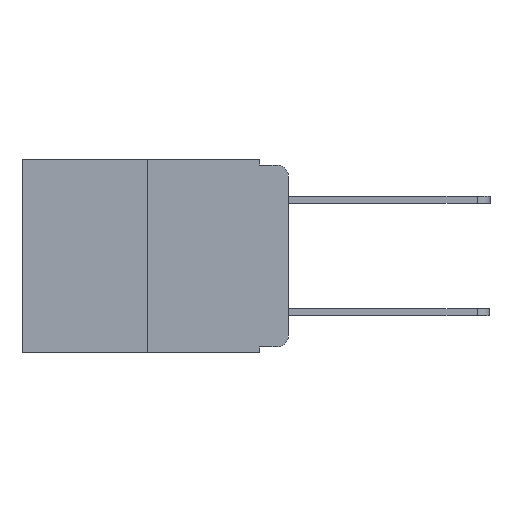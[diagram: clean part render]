
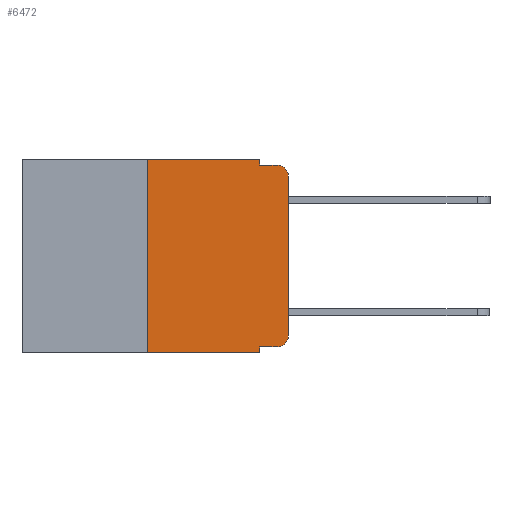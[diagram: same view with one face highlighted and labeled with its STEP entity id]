
A CAD part, left-side view. The second image highlights one B-rep face of the part: STEP entity #6472.
In plain terms, the highlighted planar face has unit normal (-1, 0, 0).
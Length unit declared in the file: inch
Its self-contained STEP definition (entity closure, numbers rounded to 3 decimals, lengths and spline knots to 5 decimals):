
#864 = EDGE_CURVE ( 'NONE', #1789, #5120, #11651, .T. ) ;
#1062 = AXIS2_PLACEMENT_3D ( 'NONE', #12072, #8657, #2610 ) ;
#1295 = ORIENTED_EDGE ( 'NONE', *, *, #1380, .F. ) ;
#1339 = DIRECTION ( 'NONE',  ( 0., -1., 0. ) ) ;
#1380 = EDGE_CURVE ( 'NONE', #1460, #12300, #2654, .T. ) ;
#1411 = ORIENTED_EDGE ( 'NONE', *, *, #11492, .F. ) ;
#1416 = VECTOR ( 'NONE', #6540, 39.37008 ) ;
#1460 = VERTEX_POINT ( 'NONE', #9998 ) ;
#1789 = VERTEX_POINT ( 'NONE', #4084 ) ;
#1919 = ORIENTED_EDGE ( 'NONE', *, *, #5005, .T. ) ;
#2190 = CARTESIAN_POINT ( 'NONE',  ( 0., 0.473, -0.343 ) ) ;
#2516 = ORIENTED_EDGE ( 'NONE', *, *, #864, .F. ) ;
#2531 = DIRECTION ( 'NONE',  ( 0., 0., -1. ) ) ;
#2559 = CIRCLE ( 'NONE', #4141, 0.02 ) ;
#2595 = LINE ( 'NONE', #4048, #12362 ) ;
#2610 = DIRECTION ( 'NONE',  ( 0., 0., -1. ) ) ;
#2654 = LINE ( 'NONE', #3460, #10198 ) ;
#2834 = DIRECTION ( 'NONE',  ( -1., 0., 0. ) ) ;
#2876 = ORIENTED_EDGE ( 'NONE', *, *, #6896, .F. ) ;
#2973 = CARTESIAN_POINT ( 'NONE',  ( 0., 0.051, -0.333 ) ) ;
#3060 = EDGE_LOOP ( 'NONE', ( #8102, #8276, #1411, #3928, #2516, #2876, #1919, #1295, #9697, #3832 ) ) ;
#3409 = DIRECTION ( 'NONE',  ( -1., 0., 0. ) ) ;
#3460 = CARTESIAN_POINT ( 'NONE',  ( 0., 0.051, 0. ) ) ;
#3470 = CARTESIAN_POINT ( 'NONE',  ( 0., 0.473, 0. ) ) ;
#3713 = EDGE_CURVE ( 'NONE', #4164, #11269, #2595, .T. ) ;
#3767 = VERTEX_POINT ( 'NONE', #9018 ) ;
#3832 = ORIENTED_EDGE ( 'NONE', *, *, #10726, .T. ) ;
#3855 = VERTEX_POINT ( 'NONE', #4547 ) ;
#3928 = ORIENTED_EDGE ( 'NONE', *, *, #8983, .F. ) ;
#4048 = CARTESIAN_POINT ( 'NONE',  ( 0., 0., 0. ) ) ;
#4082 = CIRCLE ( 'NONE', #11139, 0.02 ) ;
#4084 = CARTESIAN_POINT ( 'NONE',  ( 0., 0.25, 0. ) ) ;
#4141 = AXIS2_PLACEMENT_3D ( 'NONE', #9347, #3409, #10235 ) ;
#4164 = VERTEX_POINT ( 'NONE', #12437 ) ;
#4203 = LINE ( 'NONE', #8589, #9129 ) ;
#4547 = CARTESIAN_POINT ( 'NONE',  ( 0., 0.051, -0.01 ) ) ;
#4631 = LINE ( 'NONE', #2190, #9756 ) ;
#4725 = LINE ( 'NONE', #8410, #7398 ) ;
#5005 = EDGE_CURVE ( 'NONE', #10912, #12300, #4631, .T. ) ;
#5120 = VERTEX_POINT ( 'NONE', #8493 ) ;
#5565 = LINE ( 'NONE', #2973, #10818 ) ;
#5876 = FACE_OUTER_BOUND ( 'NONE', #3060, .T. ) ;
#5927 = VERTEX_POINT ( 'NONE', #8997 ) ;
#6472 = ADVANCED_FACE ( 'NONE', ( #5876 ), #7709, .F. ) ;
#6540 = DIRECTION ( 'NONE',  ( 0., -1., 0. ) ) ;
#6896 = EDGE_CURVE ( 'NONE', #10912, #1789, #11949, .T. ) ;
#7398 = VECTOR ( 'NONE', #1339, 39.37008 ) ;
#7470 = DIRECTION ( 'NONE',  ( 0., 0., 1. ) ) ;
#7475 = DIRECTION ( 'NONE',  ( 0., 0., 1. ) ) ;
#7709 = PLANE ( 'NONE',  #1062 ) ;
#8102 = ORIENTED_EDGE ( 'NONE', *, *, #3713, .T. ) ;
#8125 = CARTESIAN_POINT ( 'NONE',  ( 0., 0., -0.03 ) ) ;
#8269 = DIRECTION ( 'NONE',  ( 0., -1., 0. ) ) ;
#8276 = ORIENTED_EDGE ( 'NONE', *, *, #11113, .T. ) ;
#8410 = CARTESIAN_POINT ( 'NONE',  ( 0., 0.051, -0.01 ) ) ;
#8493 = CARTESIAN_POINT ( 'NONE',  ( 0., 0.051, 0. ) ) ;
#8589 = CARTESIAN_POINT ( 'NONE',  ( 0., 0.051, 0. ) ) ;
#8643 = DIRECTION ( 'NONE',  ( 0., 0., -1. ) ) ;
#8657 = DIRECTION ( 'NONE',  ( 1., 0., 0. ) ) ;
#8859 = CARTESIAN_POINT ( 'NONE',  ( 0., 0.02, -0.03 ) ) ;
#8983 = EDGE_CURVE ( 'NONE', #5120, #3855, #4203, .T. ) ;
#8997 = CARTESIAN_POINT ( 'NONE',  ( 0., 0.02, -0.01 ) ) ;
#9018 = CARTESIAN_POINT ( 'NONE',  ( 0., 0.02, -0.333 ) ) ;
#9037 = CARTESIAN_POINT ( 'NONE',  ( 0., 0.051, -0.343 ) ) ;
#9129 = VECTOR ( 'NONE', #2531, 39.37008 ) ;
#9347 = CARTESIAN_POINT ( 'NONE',  ( 0., 0.02, -0.313 ) ) ;
#9432 = VECTOR ( 'NONE', #7475, 39.37008 ) ;
#9697 = ORIENTED_EDGE ( 'NONE', *, *, #11219, .T. ) ;
#9750 = DIRECTION ( 'NONE',  ( 0., 0., -1. ) ) ;
#9756 = VECTOR ( 'NONE', #8269, 39.37008 ) ;
#9998 = CARTESIAN_POINT ( 'NONE',  ( 0., 0.051, -0.333 ) ) ;
#10198 = VECTOR ( 'NONE', #8643, 39.37008 ) ;
#10235 = DIRECTION ( 'NONE',  ( 0., 0., -1. ) ) ;
#10726 = EDGE_CURVE ( 'NONE', #3767, #4164, #2559, .T. ) ;
#10759 = DIRECTION ( 'NONE',  ( 0., -1., 0. ) ) ;
#10818 = VECTOR ( 'NONE', #10759, 39.37008 ) ;
#10912 = VERTEX_POINT ( 'NONE', #12048 ) ;
#11113 = EDGE_CURVE ( 'NONE', #11269, #5927, #4082, .T. ) ;
#11139 = AXIS2_PLACEMENT_3D ( 'NONE', #8859, #2834, #9750 ) ;
#11219 = EDGE_CURVE ( 'NONE', #1460, #3767, #5565, .T. ) ;
#11269 = VERTEX_POINT ( 'NONE', #8125 ) ;
#11492 = EDGE_CURVE ( 'NONE', #3855, #5927, #4725, .T. ) ;
#11651 = LINE ( 'NONE', #3470, #1416 ) ;
#11876 = CARTESIAN_POINT ( 'NONE',  ( 0., 0.25, 0. ) ) ;
#11949 = LINE ( 'NONE', #11876, #9432 ) ;
#12048 = CARTESIAN_POINT ( 'NONE',  ( 0., 0.25, -0.343 ) ) ;
#12072 = CARTESIAN_POINT ( 'NONE',  ( 0., 0.473, 0. ) ) ;
#12300 = VERTEX_POINT ( 'NONE', #9037 ) ;
#12362 = VECTOR ( 'NONE', #7470, 39.37008 ) ;
#12437 = CARTESIAN_POINT ( 'NONE',  ( 0., 0., -0.313 ) ) ;
